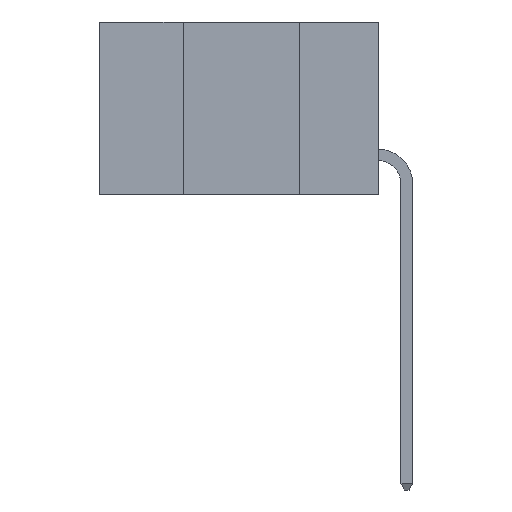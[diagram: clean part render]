
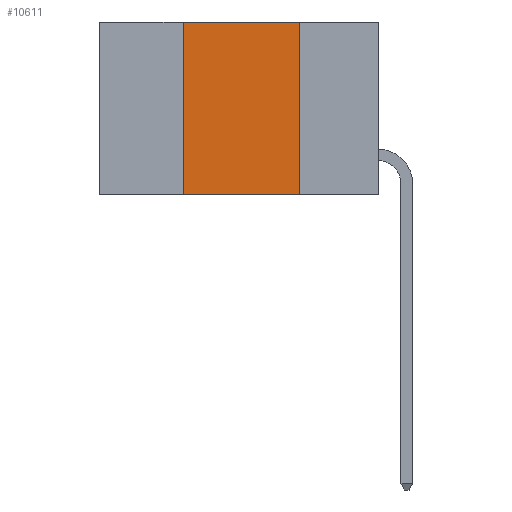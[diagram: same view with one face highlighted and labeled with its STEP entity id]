
A CAD part, left-side view. The second image highlights one B-rep face of the part: STEP entity #10611.
In plain terms, the highlighted planar face has unit normal (-1, 0, 0).
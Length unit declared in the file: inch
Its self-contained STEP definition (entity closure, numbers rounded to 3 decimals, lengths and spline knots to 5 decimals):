
#705 = VERTEX_POINT ( 'NONE', #9502 ) ;
#722 = LINE ( 'NONE', #14534, #11121 ) ;
#839 = DIRECTION ( 'NONE',  ( 1., 0., 0. ) ) ;
#958 = VECTOR ( 'NONE', #13090, 39.37008 ) ;
#1269 = DIRECTION ( 'NONE',  ( 0., 0., 1. ) ) ;
#2480 = ORIENTED_EDGE ( 'NONE', *, *, #4708, .F. ) ;
#3684 = EDGE_CURVE ( 'NONE', #21992, #18502, #722, .T. ) ;
#4708 = EDGE_CURVE ( 'NONE', #21992, #705, #22654, .T. ) ;
#6645 = CARTESIAN_POINT ( 'NONE',  ( 0., 0.6, 0. ) ) ;
#7942 = ORIENTED_EDGE ( 'NONE', *, *, #22419, .F. ) ;
#8306 = CARTESIAN_POINT ( 'NONE',  ( 0., 0.42, -0.37 ) ) ;
#9467 = DIRECTION ( 'NONE',  ( 0., 0., -1. ) ) ;
#9502 = CARTESIAN_POINT ( 'NONE',  ( 0., 0.42, 0. ) ) ;
#10365 = LINE ( 'NONE', #19167, #20100 ) ;
#10611 = ADVANCED_FACE ( 'NONE', ( #24494 ), #12523, .F. ) ;
#11121 = VECTOR ( 'NONE', #14322, 39.37008 ) ;
#12148 = EDGE_LOOP ( 'NONE', ( #7942, #23982, #2480, #13426 ) ) ;
#12523 = PLANE ( 'NONE',  #16721 ) ;
#13090 = DIRECTION ( 'NONE',  ( 0., -1., 0. ) ) ;
#13426 = ORIENTED_EDGE ( 'NONE', *, *, #3684, .T. ) ;
#14322 = DIRECTION ( 'NONE',  ( 0., -1., 0. ) ) ;
#14493 = DIRECTION ( 'NONE',  ( 0., 0., -1. ) ) ;
#14534 = CARTESIAN_POINT ( 'NONE',  ( 0., 0.6, -0.37 ) ) ;
#16513 = LINE ( 'NONE', #20813, #958 ) ;
#16721 = AXIS2_PLACEMENT_3D ( 'NONE', #6645, #839, #14493 ) ;
#17172 = CARTESIAN_POINT ( 'NONE',  ( 0., 0.17, -0.37 ) ) ;
#17541 = VECTOR ( 'NONE', #1269, 39.37008 ) ;
#18502 = VERTEX_POINT ( 'NONE', #17172 ) ;
#19167 = CARTESIAN_POINT ( 'NONE',  ( 0., 0.17, -0.37 ) ) ;
#20100 = VECTOR ( 'NONE', #9467, 39.37008 ) ;
#20341 = EDGE_CURVE ( 'NONE', #705, #21082, #16513, .T. ) ;
#20813 = CARTESIAN_POINT ( 'NONE',  ( 0., 0.6, 0. ) ) ;
#21034 = CARTESIAN_POINT ( 'NONE',  ( 0., 0.17, 0. ) ) ;
#21082 = VERTEX_POINT ( 'NONE', #21034 ) ;
#21992 = VERTEX_POINT ( 'NONE', #8306 ) ;
#22419 = EDGE_CURVE ( 'NONE', #21082, #18502, #10365, .T. ) ;
#22654 = LINE ( 'NONE', #24853, #17541 ) ;
#23982 = ORIENTED_EDGE ( 'NONE', *, *, #20341, .F. ) ;
#24494 = FACE_OUTER_BOUND ( 'NONE', #12148, .T. ) ;
#24853 = CARTESIAN_POINT ( 'NONE',  ( 0., 0.42, -0.37 ) ) ;
